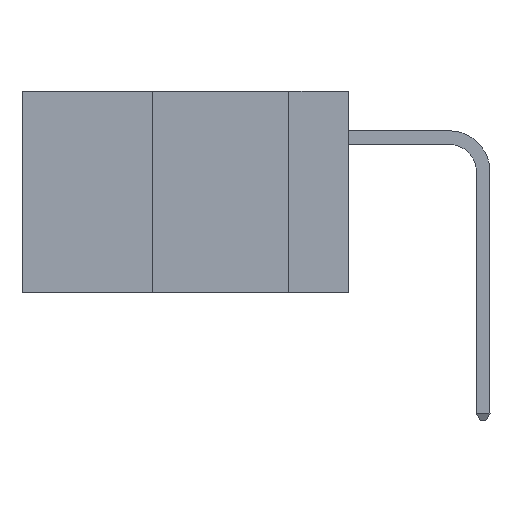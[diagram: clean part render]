
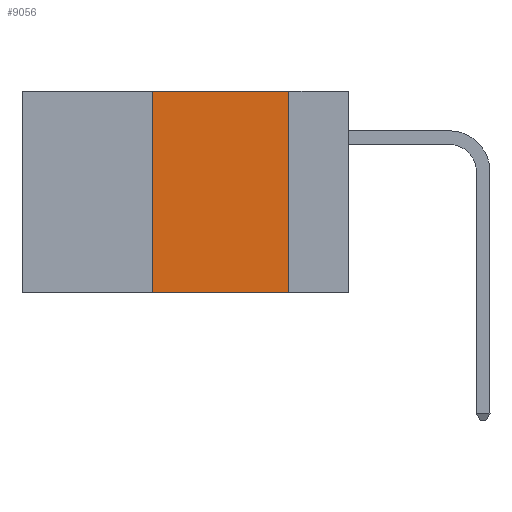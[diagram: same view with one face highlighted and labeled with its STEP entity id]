
A CAD part, left-side view. The second image highlights one B-rep face of the part: STEP entity #9056.
In plain terms, the highlighted planar face has unit normal (-1, 0, 0).
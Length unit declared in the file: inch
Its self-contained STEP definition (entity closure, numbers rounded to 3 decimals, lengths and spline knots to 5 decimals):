
#1699 = ORIENTED_EDGE ( 'NONE', *, *, #13267, .F. ) ;
#2703 = CARTESIAN_POINT ( 'NONE',  ( 0., 0.36, -0.37 ) ) ;
#2860 = EDGE_CURVE ( 'NONE', #16470, #15562, #26862, .T. ) ;
#4613 = DIRECTION ( 'NONE',  ( 1., 0., 0. ) ) ;
#6635 = DIRECTION ( 'NONE',  ( 0., 0., 1. ) ) ;
#8435 = VERTEX_POINT ( 'NONE', #19412 ) ;
#9056 = ADVANCED_FACE ( 'NONE', ( #23608 ), #20420, .F. ) ;
#10861 = CARTESIAN_POINT ( 'NONE',  ( 0., 0.11, 0. ) ) ;
#13267 = EDGE_CURVE ( 'NONE', #17311, #8435, #22623, .T. ) ;
#14043 = LINE ( 'NONE', #19487, #32225 ) ;
#15562 = VERTEX_POINT ( 'NONE', #32580 ) ;
#16470 = VERTEX_POINT ( 'NONE', #18454 ) ;
#16842 = DIRECTION ( 'NONE',  ( 0., -1., 0. ) ) ;
#17311 = VERTEX_POINT ( 'NONE', #2703 ) ;
#17907 = LINE ( 'NONE', #23379, #26645 ) ;
#18454 = CARTESIAN_POINT ( 'NONE',  ( 0., 0.11, 0. ) ) ;
#18757 = DIRECTION ( 'NONE',  ( 0., 0., -1. ) ) ;
#19175 = ORIENTED_EDGE ( 'NONE', *, *, #31166, .T. ) ;
#19412 = CARTESIAN_POINT ( 'NONE',  ( 0., 0.36, 0. ) ) ;
#19487 = CARTESIAN_POINT ( 'NONE',  ( 0., 0.6, -0.37 ) ) ;
#20238 = CARTESIAN_POINT ( 'NONE',  ( 0., 0.6, 0. ) ) ;
#20420 = PLANE ( 'NONE',  #33026 ) ;
#21479 = EDGE_CURVE ( 'NONE', #8435, #16470, #17907, .T. ) ;
#22623 = LINE ( 'NONE', #33336, #27600 ) ;
#23379 = CARTESIAN_POINT ( 'NONE',  ( 0., 0.6, 0. ) ) ;
#23608 = FACE_OUTER_BOUND ( 'NONE', #33189, .T. ) ;
#26645 = VECTOR ( 'NONE', #34085, 39.37008 ) ;
#26862 = LINE ( 'NONE', #10861, #30117 ) ;
#27242 = ORIENTED_EDGE ( 'NONE', *, *, #21479, .F. ) ;
#27600 = VECTOR ( 'NONE', #6635, 39.37008 ) ;
#29095 = ORIENTED_EDGE ( 'NONE', *, *, #2860, .F. ) ;
#30117 = VECTOR ( 'NONE', #18757, 39.37008 ) ;
#31152 = DIRECTION ( 'NONE',  ( 0., 0., -1. ) ) ;
#31166 = EDGE_CURVE ( 'NONE', #17311, #15562, #14043, .T. ) ;
#32225 = VECTOR ( 'NONE', #16842, 39.37008 ) ;
#32580 = CARTESIAN_POINT ( 'NONE',  ( 0., 0.11, -0.37 ) ) ;
#33026 = AXIS2_PLACEMENT_3D ( 'NONE', #20238, #4613, #31152 ) ;
#33189 = EDGE_LOOP ( 'NONE', ( #29095, #27242, #1699, #19175 ) ) ;
#33336 = CARTESIAN_POINT ( 'NONE',  ( 0., 0.36, 0. ) ) ;
#34085 = DIRECTION ( 'NONE',  ( 0., -1., 0. ) ) ;
